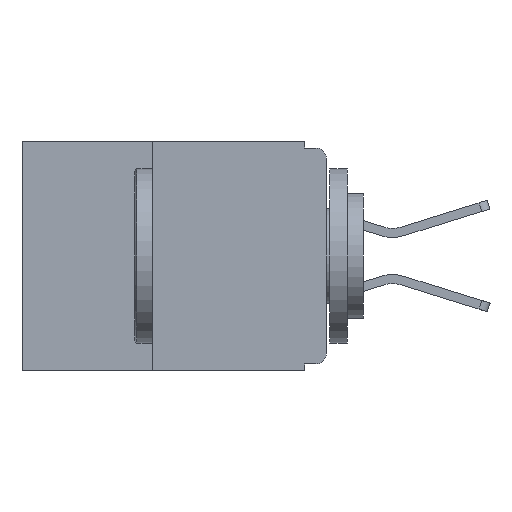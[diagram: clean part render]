
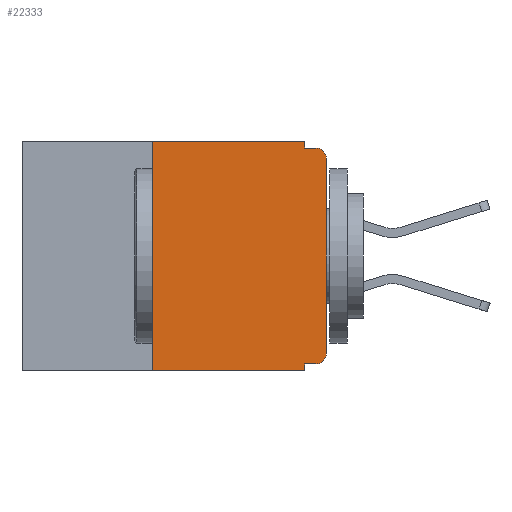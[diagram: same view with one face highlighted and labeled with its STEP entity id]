
A CAD part, left-side view. The second image highlights one B-rep face of the part: STEP entity #22333.
In plain terms, the highlighted planar face has unit normal (-1, 0, 0).
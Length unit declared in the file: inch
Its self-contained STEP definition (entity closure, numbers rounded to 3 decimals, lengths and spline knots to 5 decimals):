
#307 = DIRECTION ( 'NONE',  ( 0., 1., 0. ) ) ;
#374 = VECTOR ( 'NONE', #307, 39.37008 ) ;
#994 = VERTEX_POINT ( 'NONE', #1477 ) ;
#1038 = ORIENTED_EDGE ( 'NONE', *, *, #27841, .T. ) ;
#1477 = CARTESIAN_POINT ( 'NONE',  ( 0., 0.015, -0.32 ) ) ;
#1865 = ORIENTED_EDGE ( 'NONE', *, *, #31315, .T. ) ;
#1973 = VECTOR ( 'NONE', #13951, 39.37008 ) ;
#2098 = ORIENTED_EDGE ( 'NONE', *, *, #23404, .F. ) ;
#2546 = ORIENTED_EDGE ( 'NONE', *, *, #30390, .F. ) ;
#3388 = EDGE_CURVE ( 'NONE', #5118, #13540, #28066, .T. ) ;
#3414 = CARTESIAN_POINT ( 'NONE',  ( 0., 0.015, -0.025 ) ) ;
#3581 = ORIENTED_EDGE ( 'NONE', *, *, #12160, .F. ) ;
#3670 = DIRECTION ( 'NONE',  ( -1., 0., 0. ) ) ;
#3993 = ORIENTED_EDGE ( 'NONE', *, *, #15357, .F. ) ;
#4223 = VERTEX_POINT ( 'NONE', #23108 ) ;
#4301 = ORIENTED_EDGE ( 'NONE', *, *, #10358, .T. ) ;
#4758 = EDGE_LOOP ( 'NONE', ( #1038, #1865, #2098, #2546, #3581, #3993, #4301, #5457, #5790, #5819 ) ) ;
#5118 = VERTEX_POINT ( 'NONE', #14783 ) ;
#5138 = CARTESIAN_POINT ( 'NONE',  ( 0., 0.437, -0.33 ) ) ;
#5174 = CARTESIAN_POINT ( 'NONE',  ( 0., 0.031, -0.01 ) ) ;
#5440 = VECTOR ( 'NONE', #22834, 39.37008 ) ;
#5457 = ORIENTED_EDGE ( 'NONE', *, *, #3388, .F. ) ;
#5790 = ORIENTED_EDGE ( 'NONE', *, *, #12353, .F. ) ;
#5819 = ORIENTED_EDGE ( 'NONE', *, *, #11284, .T. ) ;
#6096 = DIRECTION ( 'NONE',  ( 0., 0., -1. ) ) ;
#6260 = AXIS2_PLACEMENT_3D ( 'NONE', #26839, #31783, #16891 ) ;
#6359 = CARTESIAN_POINT ( 'NONE',  ( 0., 0.031, 0. ) ) ;
#6431 = AXIS2_PLACEMENT_3D ( 'NONE', #18840, #3670, #21361 ) ;
#6686 = CARTESIAN_POINT ( 'NONE',  ( 0., 0.015, -0.01 ) ) ;
#6906 = DIRECTION ( 'NONE',  ( 0., 0., 1. ) ) ;
#7518 = DIRECTION ( 'NONE',  ( 0., 0., -1. ) ) ;
#8414 = CARTESIAN_POINT ( 'NONE',  ( 0., 0., -0.01 ) ) ;
#9449 = CARTESIAN_POINT ( 'NONE',  ( 0., 0.25, -0.33 ) ) ;
#10202 = VERTEX_POINT ( 'NONE', #14358 ) ;
#10358 = EDGE_CURVE ( 'NONE', #10202, #13540, #12232, .T. ) ;
#10911 = CARTESIAN_POINT ( 'NONE',  ( 0., 0., 0. ) ) ;
#11284 = EDGE_CURVE ( 'NONE', #994, #4223, #13726, .T. ) ;
#12160 = EDGE_CURVE ( 'NONE', #13506, #27988, #19496, .T. ) ;
#12232 = LINE ( 'NONE', #5138, #5440 ) ;
#12353 = EDGE_CURVE ( 'NONE', #994, #5118, #20660, .T. ) ;
#12850 = CARTESIAN_POINT ( 'NONE',  ( 0., 0.031, -0.33 ) ) ;
#13506 = VERTEX_POINT ( 'NONE', #16882 ) ;
#13540 = VERTEX_POINT ( 'NONE', #17090 ) ;
#13726 = CIRCLE ( 'NONE', #6431, 0.015 ) ;
#13951 = DIRECTION ( 'NONE',  ( 0., 0., -1. ) ) ;
#14358 = CARTESIAN_POINT ( 'NONE',  ( 0., 0.25, -0.33 ) ) ;
#14783 = CARTESIAN_POINT ( 'NONE',  ( 0., 0.031, -0.32 ) ) ;
#14967 = LINE ( 'NONE', #8414, #27485 ) ;
#15357 = EDGE_CURVE ( 'NONE', #10202, #13506, #15864, .T. ) ;
#15864 = LINE ( 'NONE', #9449, #28365 ) ;
#16882 = CARTESIAN_POINT ( 'NONE',  ( 0., 0.25, 0. ) ) ;
#16891 = DIRECTION ( 'NONE',  ( 0., 0., -1. ) ) ;
#17090 = CARTESIAN_POINT ( 'NONE',  ( 0., 0.031, -0.33 ) ) ;
#17394 = CARTESIAN_POINT ( 'NONE',  ( 0., 0.437, 0. ) ) ;
#17633 = VECTOR ( 'NONE', #25974, 39.37008 ) ;
#18333 = DIRECTION ( 'NONE',  ( 0., -1., 0. ) ) ;
#18606 = CARTESIAN_POINT ( 'NONE',  ( 0., 0., -0.025 ) ) ;
#18624 = VERTEX_POINT ( 'NONE', #5174 ) ;
#18702 = VECTOR ( 'NONE', #19892, 39.37008 ) ;
#18840 = CARTESIAN_POINT ( 'NONE',  ( 0., 0.015, -0.305 ) ) ;
#19496 = LINE ( 'NONE', #17394, #18702 ) ;
#19892 = DIRECTION ( 'NONE',  ( 0., -1., 0. ) ) ;
#20564 = LINE ( 'NONE', #27442, #31448 ) ;
#20660 = LINE ( 'NONE', #30546, #374 ) ;
#21121 = DIRECTION ( 'NONE',  ( -1., 0., 0. ) ) ;
#21361 = DIRECTION ( 'NONE',  ( 0., 0., -1. ) ) ;
#22074 = FACE_OUTER_BOUND ( 'NONE', #4758, .T. ) ;
#22333 = ADVANCED_FACE ( 'NONE', ( #22074 ), #31677, .F. ) ;
#22834 = DIRECTION ( 'NONE',  ( 0., -1., 0. ) ) ;
#23108 = CARTESIAN_POINT ( 'NONE',  ( 0., 0., -0.305 ) ) ;
#23404 = EDGE_CURVE ( 'NONE', #18624, #27171, #14967, .T. ) ;
#24259 = LINE ( 'NONE', #10911, #17633 ) ;
#24404 = AXIS2_PLACEMENT_3D ( 'NONE', #3414, #21121, #6096 ) ;
#25758 = VERTEX_POINT ( 'NONE', #18606 ) ;
#25974 = DIRECTION ( 'NONE',  ( 0., 0., 1. ) ) ;
#26839 = CARTESIAN_POINT ( 'NONE',  ( 0., 0.437, 0. ) ) ;
#27171 = VERTEX_POINT ( 'NONE', #6686 ) ;
#27442 = CARTESIAN_POINT ( 'NONE',  ( 0., 0.031, 0. ) ) ;
#27485 = VECTOR ( 'NONE', #18333, 39.37008 ) ;
#27841 = EDGE_CURVE ( 'NONE', #4223, #25758, #24259, .T. ) ;
#27988 = VERTEX_POINT ( 'NONE', #6359 ) ;
#28066 = LINE ( 'NONE', #12850, #1973 ) ;
#28365 = VECTOR ( 'NONE', #6906, 39.37008 ) ;
#29858 = CIRCLE ( 'NONE', #24404, 0.015 ) ;
#30390 = EDGE_CURVE ( 'NONE', #27988, #18624, #20564, .T. ) ;
#30546 = CARTESIAN_POINT ( 'NONE',  ( 0., 0., -0.32 ) ) ;
#31315 = EDGE_CURVE ( 'NONE', #25758, #27171, #29858, .T. ) ;
#31448 = VECTOR ( 'NONE', #7518, 39.37008 ) ;
#31677 = PLANE ( 'NONE',  #6260 ) ;
#31783 = DIRECTION ( 'NONE',  ( 1., 0., 0. ) ) ;
